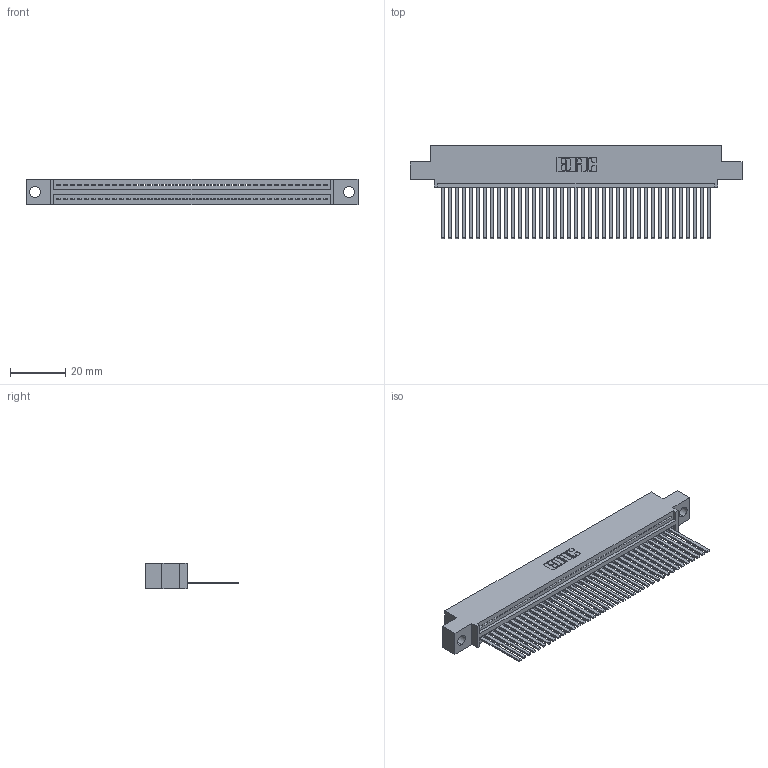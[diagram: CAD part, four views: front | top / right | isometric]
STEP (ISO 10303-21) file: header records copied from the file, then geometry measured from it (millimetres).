
FILE_DESCRIPTION (( 'STEP AP203' ), '1' );
FILE_NAME ('345-039-544-404.STEP', '2018-09-04T23:41:30', ( '' ), ( '' ), 'SwSTEP 2.0', 'SolidWorks 2016', '' );
FILE_SCHEMA (( 'CONFIG_CONTROL_DESIGN' ));
Length unit declared in the file: inch
Products named in the file (3): 345 Part_0.110 Offset - 0.156 Dia-TH; 345-292-001_345-293-144; 345-039-544-404
Assembly tree (40 placements, depth 2):
  345-039-544-404
    345 Part_0.110 Offset - 0.156 Dia-TH
    345-292-001_345-293-144  x39
Bounding box: 120.27 x 33.96 x 9.4 mm (x, y, z)
Volume: 11689.1 mm3; surface area: 16739.7 mm2
Topology: 40 solids, 40 shells, 2158 faces, 6515 edges, 4290 vertices
Faces by surface type: plane 1488, cylinder 670
Entity records: 29707 total; most frequent: CARTESIAN_POINT 5153, ORIENTED_EDGE 5126, DIRECTION 4501, EDGE_CURVE 2563, VECTOR 2279, LINE 2279, VERTEX_POINT 1706, AXIS2_PLACEMENT_3D 1111
